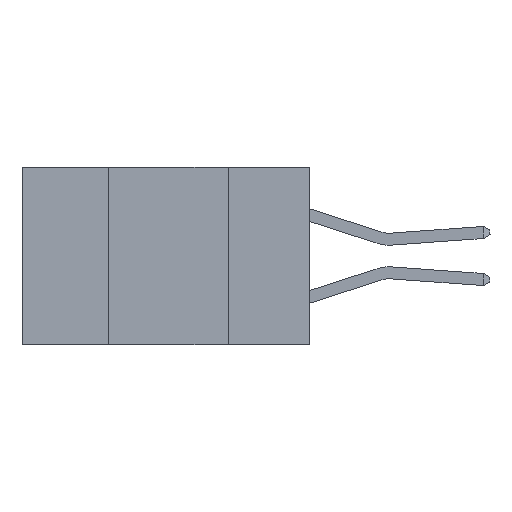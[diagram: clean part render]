
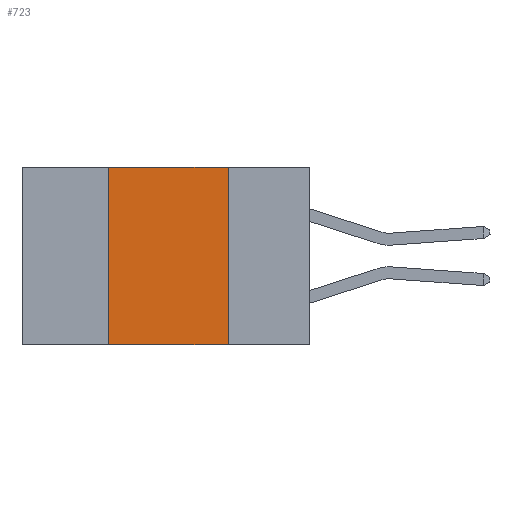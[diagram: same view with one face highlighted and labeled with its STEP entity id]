
A CAD part, left-side view. The second image highlights one B-rep face of the part: STEP entity #723.
In plain terms, the highlighted planar face has unit normal (-1, 0, 0).
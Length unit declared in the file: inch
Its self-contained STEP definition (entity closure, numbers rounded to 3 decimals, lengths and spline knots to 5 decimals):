
#53 = CARTESIAN_POINT ( 'NONE',  ( 0., 0.17, -0.37 ) ) ;
#563 = LINE ( 'NONE', #9730, #1380 ) ;
#723 = ADVANCED_FACE ( 'NONE', ( #13405 ), #9860, .F. ) ;
#952 = VERTEX_POINT ( 'NONE', #14323 ) ;
#1380 = VECTOR ( 'NONE', #11036, 39.37008 ) ;
#1381 = LINE ( 'NONE', #10790, #7822 ) ;
#1553 = CARTESIAN_POINT ( 'NONE',  ( 0., 0.42, -0.37 ) ) ;
#2405 = DIRECTION ( 'NONE',  ( 0., -1., 0. ) ) ;
#2923 = DIRECTION ( 'NONE',  ( 0., 0., -1. ) ) ;
#3240 = DIRECTION ( 'NONE',  ( 1., 0., 0. ) ) ;
#3357 = DIRECTION ( 'NONE',  ( 0., -1., 0. ) ) ;
#3547 = VECTOR ( 'NONE', #2405, 39.37008 ) ;
#4676 = CARTESIAN_POINT ( 'NONE',  ( 0., 0.6, 0. ) ) ;
#4765 = ORIENTED_EDGE ( 'NONE', *, *, #4805, .F. ) ;
#4805 = EDGE_CURVE ( 'NONE', #8559, #952, #1381, .T. ) ;
#5040 = ORIENTED_EDGE ( 'NONE', *, *, #12162, .F. ) ;
#5916 = ORIENTED_EDGE ( 'NONE', *, *, #15384, .T. ) ;
#6288 = VERTEX_POINT ( 'NONE', #14758 ) ;
#7002 = EDGE_CURVE ( 'NONE', #952, #6288, #13827, .T. ) ;
#7822 = VECTOR ( 'NONE', #16636, 39.37008 ) ;
#8559 = VERTEX_POINT ( 'NONE', #1553 ) ;
#9730 = CARTESIAN_POINT ( 'NONE',  ( 0., 0.17, 0. ) ) ;
#9860 = PLANE ( 'NONE',  #12281 ) ;
#10064 = CARTESIAN_POINT ( 'NONE',  ( 0., 0.6, 0. ) ) ;
#10790 = CARTESIAN_POINT ( 'NONE',  ( 0., 0.42, 0. ) ) ;
#11036 = DIRECTION ( 'NONE',  ( 0., 0., -1. ) ) ;
#12162 = EDGE_CURVE ( 'NONE', #6288, #12443, #563, .T. ) ;
#12281 = AXIS2_PLACEMENT_3D ( 'NONE', #4676, #3240, #2923 ) ;
#12443 = VERTEX_POINT ( 'NONE', #53 ) ;
#13405 = FACE_OUTER_BOUND ( 'NONE', #15942, .T. ) ;
#13827 = LINE ( 'NONE', #10064, #3547 ) ;
#14323 = CARTESIAN_POINT ( 'NONE',  ( 0., 0.42, 0. ) ) ;
#14758 = CARTESIAN_POINT ( 'NONE',  ( 0., 0.17, 0. ) ) ;
#14971 = CARTESIAN_POINT ( 'NONE',  ( 0., 0.6, -0.37 ) ) ;
#15163 = ORIENTED_EDGE ( 'NONE', *, *, #7002, .F. ) ;
#15384 = EDGE_CURVE ( 'NONE', #8559, #12443, #15921, .T. ) ;
#15540 = VECTOR ( 'NONE', #3357, 39.37008 ) ;
#15921 = LINE ( 'NONE', #14971, #15540 ) ;
#15942 = EDGE_LOOP ( 'NONE', ( #5040, #15163, #4765, #5916 ) ) ;
#16636 = DIRECTION ( 'NONE',  ( 0., 0., 1. ) ) ;
